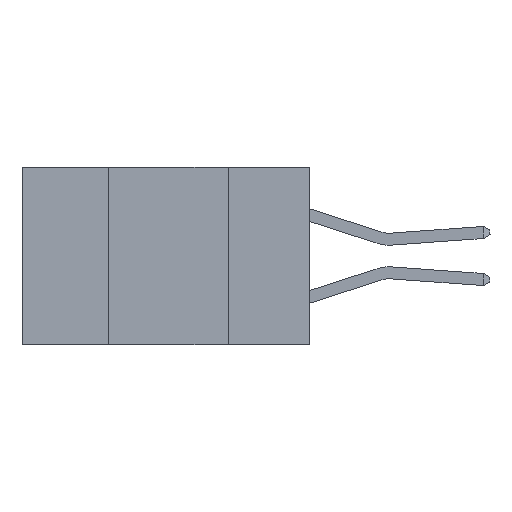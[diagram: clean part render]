
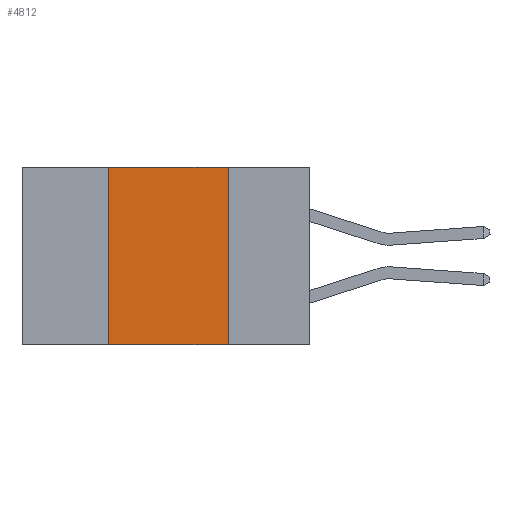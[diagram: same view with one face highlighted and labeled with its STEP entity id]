
A CAD part, left-side view. The second image highlights one B-rep face of the part: STEP entity #4812.
In plain terms, the highlighted planar face has unit normal (-1, 0, 0).
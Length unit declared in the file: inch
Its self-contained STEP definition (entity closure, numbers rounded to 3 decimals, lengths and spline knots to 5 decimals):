
#102 = CARTESIAN_POINT ( 'NONE',  ( 0., 0.6, 0. ) ) ;
#175 = CARTESIAN_POINT ( 'NONE',  ( 0., 0.6, 0. ) ) ;
#376 = LINE ( 'NONE', #4359, #11989 ) ;
#1152 = LINE ( 'NONE', #175, #11823 ) ;
#1662 = PLANE ( 'NONE',  #2153 ) ;
#1836 = EDGE_CURVE ( 'NONE', #6831, #5462, #5365, .T. ) ;
#2153 = AXIS2_PLACEMENT_3D ( 'NONE', #102, #3091, #9969 ) ;
#2345 = DIRECTION ( 'NONE',  ( 0., 0., -1. ) ) ;
#3091 = DIRECTION ( 'NONE',  ( 1., 0., 0. ) ) ;
#4292 = DIRECTION ( 'NONE',  ( 0., 0., 1. ) ) ;
#4359 = CARTESIAN_POINT ( 'NONE',  ( 0., 0.42, -0.37 ) ) ;
#4664 = VERTEX_POINT ( 'NONE', #6395 ) ;
#4812 = ADVANCED_FACE ( 'NONE', ( #10614 ), #1662, .F. ) ;
#5158 = VECTOR ( 'NONE', #12820, 39.37008 ) ;
#5365 = LINE ( 'NONE', #7218, #6963 ) ;
#5462 = VERTEX_POINT ( 'NONE', #6300 ) ;
#6300 = CARTESIAN_POINT ( 'NONE',  ( 0., 0.17, -0.37 ) ) ;
#6395 = CARTESIAN_POINT ( 'NONE',  ( 0., 0.42, 0. ) ) ;
#6687 = CARTESIAN_POINT ( 'NONE',  ( 0., 0.17, 0. ) ) ;
#6831 = VERTEX_POINT ( 'NONE', #6687 ) ;
#6963 = VECTOR ( 'NONE', #2345, 39.37008 ) ;
#7130 = LINE ( 'NONE', #11849, #5158 ) ;
#7190 = DIRECTION ( 'NONE',  ( 0., -1., 0. ) ) ;
#7218 = CARTESIAN_POINT ( 'NONE',  ( 0., 0.17, -0.37 ) ) ;
#7804 = ORIENTED_EDGE ( 'NONE', *, *, #8898, .F. ) ;
#8594 = CARTESIAN_POINT ( 'NONE',  ( 0., 0.42, -0.37 ) ) ;
#8838 = EDGE_LOOP ( 'NONE', ( #9183, #11591, #7804, #12082 ) ) ;
#8898 = EDGE_CURVE ( 'NONE', #11313, #4664, #376, .T. ) ;
#9183 = ORIENTED_EDGE ( 'NONE', *, *, #1836, .F. ) ;
#9969 = DIRECTION ( 'NONE',  ( 0., 0., -1. ) ) ;
#10531 = EDGE_CURVE ( 'NONE', #11313, #5462, #7130, .T. ) ;
#10614 = FACE_OUTER_BOUND ( 'NONE', #8838, .T. ) ;
#10769 = EDGE_CURVE ( 'NONE', #4664, #6831, #1152, .T. ) ;
#11313 = VERTEX_POINT ( 'NONE', #8594 ) ;
#11591 = ORIENTED_EDGE ( 'NONE', *, *, #10769, .F. ) ;
#11823 = VECTOR ( 'NONE', #7190, 39.37008 ) ;
#11849 = CARTESIAN_POINT ( 'NONE',  ( 0., 0.6, -0.37 ) ) ;
#11989 = VECTOR ( 'NONE', #4292, 39.37008 ) ;
#12082 = ORIENTED_EDGE ( 'NONE', *, *, #10531, .T. ) ;
#12820 = DIRECTION ( 'NONE',  ( 0., -1., 0. ) ) ;
